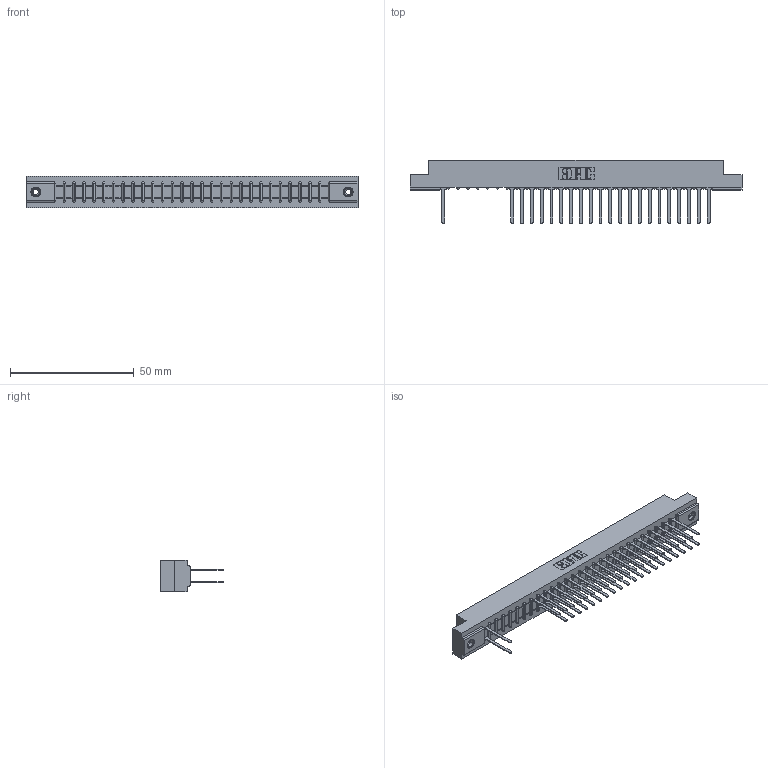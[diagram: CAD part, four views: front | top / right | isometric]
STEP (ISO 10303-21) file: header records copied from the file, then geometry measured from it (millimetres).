
FILE_DESCRIPTION (( 'STEP AP203' ), '1' );
FILE_NAME ('307-056-542-208.STEP', '2018-08-06T06:52:47', ( '' ), ( '' ), 'SwSTEP 2.0', 'SolidWorks 2016', '' );
FILE_SCHEMA (( 'CONFIG_CONTROL_DESIGN' ));
Length unit declared in the file: inch
Products named in the file (4): 345-250-001_345-250-003-102; 307-056-542-208; 307 Part_.156 Dia Mounting Holes; 307-290-001_542
Assembly tree (46 placements, depth 2):
  307-056-542-208
    307 Part_.156 Dia Mounting Holes
    307-290-001_542  x43
    345-250-001_345-250-003-102  x2
Bounding box: 133.96 x 25.43 x 12.7 mm (x, y, z)
Volume: 14135.2 mm3; surface area: 16865.9 mm2
Topology: 46 solids, 46 shells, 2315 faces, 6465 edges, 4166 vertices
Faces by surface type: plane 1513, cylinder 728, sphere 58, cone 12, torus 4
Entity records: 27363 total; most frequent: CARTESIAN_POINT 4518, ORIENTED_EDGE 4482, DIRECTION 4427, EDGE_CURVE 2241, VECTOR 1713, LINE 1713, VERTEX_POINT 1448, AXIS2_PLACEMENT_3D 1357
